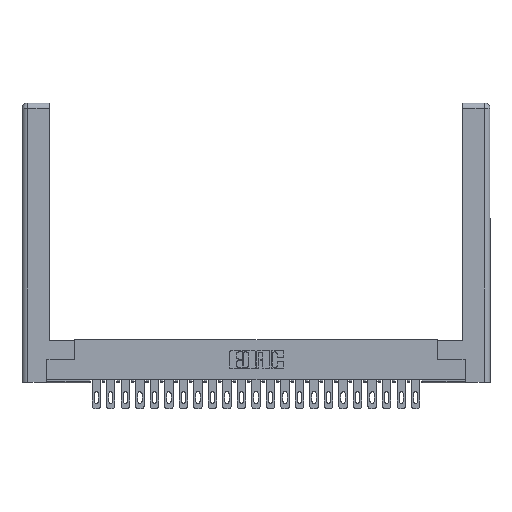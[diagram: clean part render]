
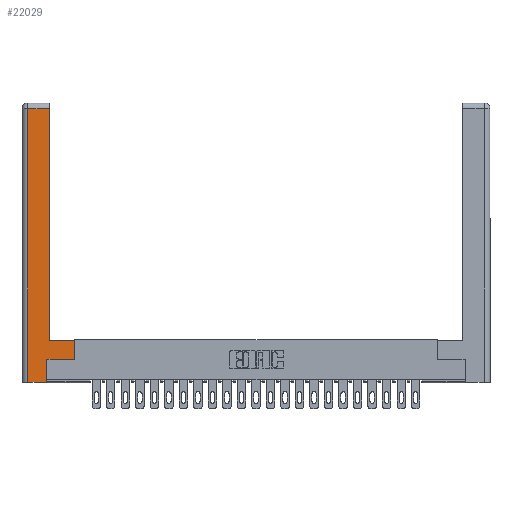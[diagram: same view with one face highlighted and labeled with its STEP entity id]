
A CAD part, top view. The second image highlights one B-rep face of the part: STEP entity #22029.
In plain terms, the highlighted planar face has unit normal (0, 0, 1).
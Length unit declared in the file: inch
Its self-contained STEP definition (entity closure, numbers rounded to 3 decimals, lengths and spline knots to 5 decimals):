
#440 = LINE ( 'NONE', #26929, #24241 ) ;
#604 = ORIENTED_EDGE ( 'NONE', *, *, #14680, .T. ) ;
#1705 = DIRECTION ( 'NONE',  ( -1., 0., 0. ) ) ;
#3848 = VECTOR ( 'NONE', #27216, 39.37008 ) ;
#4004 = DIRECTION ( 'NONE',  ( 0., 1., 0. ) ) ;
#4356 = EDGE_LOOP ( 'NONE', ( #14129, #7084, #20360, #6816, #13252, #604, #18473, #21356 ) ) ;
#4601 = VECTOR ( 'NONE', #5031, 39.37008 ) ;
#5031 = DIRECTION ( 'NONE',  ( 0., 1., 0. ) ) ;
#5322 = CARTESIAN_POINT ( 'NONE',  ( 0.565, 0.45, 0. ) ) ;
#5840 = DIRECTION ( 'NONE',  ( 0., -1., 0. ) ) ;
#6201 = LINE ( 'NONE', #25781, #13435 ) ;
#6816 = ORIENTED_EDGE ( 'NONE', *, *, #17105, .T. ) ;
#7084 = ORIENTED_EDGE ( 'NONE', *, *, #20654, .T. ) ;
#7218 = CARTESIAN_POINT ( 'NONE',  ( 0.565, 0.245, 0. ) ) ;
#7852 = CARTESIAN_POINT ( 'NONE',  ( 0., 0., 0. ) ) ;
#9462 = LINE ( 'NONE', #13471, #10925 ) ;
#10732 = LINE ( 'NONE', #14444, #4601 ) ;
#10925 = VECTOR ( 'NONE', #29595, 39.37008 ) ;
#11427 = AXIS2_PLACEMENT_3D ( 'NONE', #7852, #14650, #23804 ) ;
#12843 = VERTEX_POINT ( 'NONE', #28109 ) ;
#13156 = DIRECTION ( 'NONE',  ( -1., 0., 0. ) ) ;
#13252 = ORIENTED_EDGE ( 'NONE', *, *, #25321, .T. ) ;
#13435 = VECTOR ( 'NONE', #14625, 39.37008 ) ;
#13471 = CARTESIAN_POINT ( 'NONE',  ( 0.265, 0., 0. ) ) ;
#13513 = CARTESIAN_POINT ( 'NONE',  ( 0.565, 0.45, 0. ) ) ;
#13537 = CARTESIAN_POINT ( 'NONE',  ( 0.565, 0.245, 0. ) ) ;
#14129 = ORIENTED_EDGE ( 'NONE', *, *, #14234, .T. ) ;
#14234 = EDGE_CURVE ( 'NONE', #20023, #16802, #10732, .T. ) ;
#14444 = CARTESIAN_POINT ( 'NONE',  ( 0.295, 3., 0. ) ) ;
#14625 = DIRECTION ( 'NONE',  ( 0., 1., 0. ) ) ;
#14650 = DIRECTION ( 'NONE',  ( 0., 0., -1. ) ) ;
#14680 = EDGE_CURVE ( 'NONE', #18248, #16375, #16161, .T. ) ;
#15664 = CARTESIAN_POINT ( 'NONE',  ( 0.295, 0.45, 0. ) ) ;
#16161 = LINE ( 'NONE', #13537, #3848 ) ;
#16261 = CARTESIAN_POINT ( 'NONE',  ( 0.0615, 0., 0. ) ) ;
#16375 = VERTEX_POINT ( 'NONE', #7218 ) ;
#16802 = VERTEX_POINT ( 'NONE', #18275 ) ;
#17105 = EDGE_CURVE ( 'NONE', #25606, #28183, #9462, .T. ) ;
#17858 = VECTOR ( 'NONE', #4004, 39.37008 ) ;
#18248 = VERTEX_POINT ( 'NONE', #21054 ) ;
#18275 = CARTESIAN_POINT ( 'NONE',  ( 0.295, 2.94, 0. ) ) ;
#18473 = ORIENTED_EDGE ( 'NONE', *, *, #20331, .T. ) ;
#20023 = VERTEX_POINT ( 'NONE', #15664 ) ;
#20061 = CARTESIAN_POINT ( 'NONE',  ( 0.0615, 2.94, 0. ) ) ;
#20331 = EDGE_CURVE ( 'NONE', #16375, #22110, #20342, .T. ) ;
#20342 = LINE ( 'NONE', #13513, #17858 ) ;
#20360 = ORIENTED_EDGE ( 'NONE', *, *, #22228, .T. ) ;
#20654 = EDGE_CURVE ( 'NONE', #16802, #12843, #23523, .T. ) ;
#21054 = CARTESIAN_POINT ( 'NONE',  ( 0.265, 0.245, 0. ) ) ;
#21356 = ORIENTED_EDGE ( 'NONE', *, *, #21526, .T. ) ;
#21526 = EDGE_CURVE ( 'NONE', #22110, #20023, #440, .T. ) ;
#22029 = ADVANCED_FACE ( 'NONE', ( #29652 ), #28439, .F. ) ;
#22110 = VERTEX_POINT ( 'NONE', #5322 ) ;
#22228 = EDGE_CURVE ( 'NONE', #12843, #25606, #23829, .T. ) ;
#23523 = LINE ( 'NONE', #20061, #26763 ) ;
#23804 = DIRECTION ( 'NONE',  ( -1., 0., 0. ) ) ;
#23829 = LINE ( 'NONE', #26817, #25291 ) ;
#24060 = CARTESIAN_POINT ( 'NONE',  ( 0.265, 0., 0. ) ) ;
#24241 = VECTOR ( 'NONE', #13156, 39.37008 ) ;
#25291 = VECTOR ( 'NONE', #5840, 39.37008 ) ;
#25321 = EDGE_CURVE ( 'NONE', #28183, #18248, #6201, .T. ) ;
#25606 = VERTEX_POINT ( 'NONE', #16261 ) ;
#25781 = CARTESIAN_POINT ( 'NONE',  ( 0.265, 0.245, 0. ) ) ;
#26763 = VECTOR ( 'NONE', #1705, 39.37008 ) ;
#26817 = CARTESIAN_POINT ( 'NONE',  ( 0.0615, 0., 0. ) ) ;
#26929 = CARTESIAN_POINT ( 'NONE',  ( 0.295, 0.45, 0. ) ) ;
#27216 = DIRECTION ( 'NONE',  ( 1., 0., 0. ) ) ;
#28109 = CARTESIAN_POINT ( 'NONE',  ( 0.0615, 2.94, 0. ) ) ;
#28183 = VERTEX_POINT ( 'NONE', #24060 ) ;
#28439 = PLANE ( 'NONE',  #11427 ) ;
#29595 = DIRECTION ( 'NONE',  ( 1., 0., 0. ) ) ;
#29652 = FACE_OUTER_BOUND ( 'NONE', #4356, .T. ) ;
